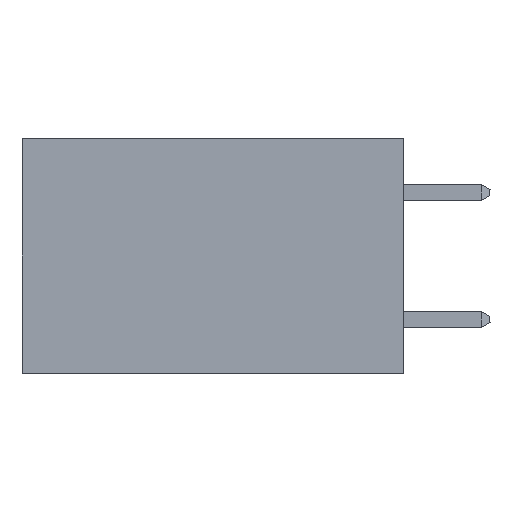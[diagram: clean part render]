
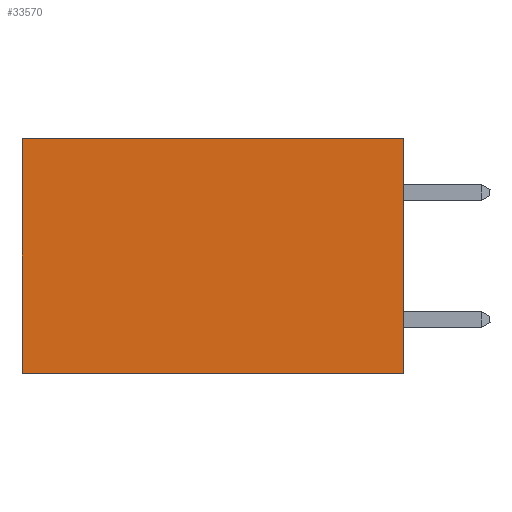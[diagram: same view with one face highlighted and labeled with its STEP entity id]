
A CAD part, left-side view. The second image highlights one B-rep face of the part: STEP entity #33570.
In plain terms, the highlighted planar face has unit normal (-1, 0, 0).
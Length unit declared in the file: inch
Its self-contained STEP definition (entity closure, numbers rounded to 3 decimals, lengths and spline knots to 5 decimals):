
#1499 = CARTESIAN_POINT ( 'NONE',  ( 0.2875, 0.6, -0.37 ) ) ;
#2034 = LINE ( 'NONE', #11901, #15079 ) ;
#2124 = VERTEX_POINT ( 'NONE', #1499 ) ;
#4297 = EDGE_CURVE ( 'NONE', #29286, #14780, #29634, .T. ) ;
#5034 = DIRECTION ( 'NONE',  ( 0., 0., -1. ) ) ;
#5157 = CARTESIAN_POINT ( 'NONE',  ( 0.2875, 0., 0. ) ) ;
#5453 = VECTOR ( 'NONE', #18975, 39.37008 ) ;
#8531 = ORIENTED_EDGE ( 'NONE', *, *, #15905, .F. ) ;
#10272 = CARTESIAN_POINT ( 'NONE',  ( 0.2875, 0., 0. ) ) ;
#11901 = CARTESIAN_POINT ( 'NONE',  ( 0.2875, 0., -0.37 ) ) ;
#11990 = ORIENTED_EDGE ( 'NONE', *, *, #32329, .T. ) ;
#13068 = ORIENTED_EDGE ( 'NONE', *, *, #14352, .F. ) ;
#13270 = DIRECTION ( 'NONE',  ( 0., 0., -1. ) ) ;
#14221 = CARTESIAN_POINT ( 'NONE',  ( 0.2875, 0., 0. ) ) ;
#14352 = EDGE_CURVE ( 'NONE', #35396, #2124, #2034, .T. ) ;
#14721 = LINE ( 'NONE', #28030, #17080 ) ;
#14780 = VERTEX_POINT ( 'NONE', #20277 ) ;
#15079 = VECTOR ( 'NONE', #15271, 39.37008 ) ;
#15080 = FACE_OUTER_BOUND ( 'NONE', #19444, .T. ) ;
#15271 = DIRECTION ( 'NONE',  ( 0., 1., 0. ) ) ;
#15905 = EDGE_CURVE ( 'NONE', #29286, #35396, #16830, .T. ) ;
#16083 = AXIS2_PLACEMENT_3D ( 'NONE', #5157, #25803, #5034 ) ;
#16830 = LINE ( 'NONE', #30562, #29834 ) ;
#17080 = VECTOR ( 'NONE', #13270, 39.37008 ) ;
#18975 = DIRECTION ( 'NONE',  ( 0., 1., 0. ) ) ;
#19444 = EDGE_LOOP ( 'NONE', ( #11990, #13068, #8531, #30854 ) ) ;
#20277 = CARTESIAN_POINT ( 'NONE',  ( 0.2875, 0.6, 0. ) ) ;
#20896 = CARTESIAN_POINT ( 'NONE',  ( 0.2875, 0., -0.37 ) ) ;
#24557 = DIRECTION ( 'NONE',  ( 0., 0., -1. ) ) ;
#25803 = DIRECTION ( 'NONE',  ( 1., 0., 0. ) ) ;
#28030 = CARTESIAN_POINT ( 'NONE',  ( 0.2875, 0.6, 0. ) ) ;
#29286 = VERTEX_POINT ( 'NONE', #14221 ) ;
#29634 = LINE ( 'NONE', #10272, #5453 ) ;
#29834 = VECTOR ( 'NONE', #24557, 39.37008 ) ;
#30562 = CARTESIAN_POINT ( 'NONE',  ( 0.2875, 0., 0. ) ) ;
#30854 = ORIENTED_EDGE ( 'NONE', *, *, #4297, .T. ) ;
#30911 = PLANE ( 'NONE',  #16083 ) ;
#32329 = EDGE_CURVE ( 'NONE', #14780, #2124, #14721, .T. ) ;
#33570 = ADVANCED_FACE ( 'NONE', ( #15080 ), #30911, .F. ) ;
#35396 = VERTEX_POINT ( 'NONE', #20896 ) ;
